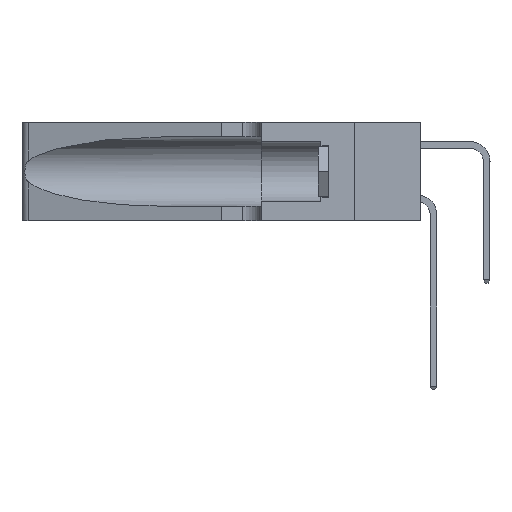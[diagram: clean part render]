
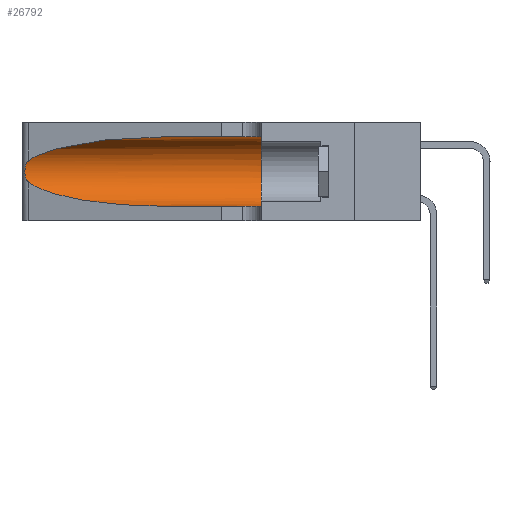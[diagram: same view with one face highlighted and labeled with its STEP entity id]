
A CAD part, left-side view. The second image highlights one B-rep face of the part: STEP entity #26792.
In plain terms, the highlighted cylindrical face has radius 3.308 mm (diameter 6.617 mm), a partial arc.
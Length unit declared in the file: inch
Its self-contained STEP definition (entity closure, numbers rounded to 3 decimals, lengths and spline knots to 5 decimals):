
#36 = EDGE_CURVE ( 'NONE', #20641, #6997, #20732, .T. ) ;
#122 =( BOUNDED_CURVE ( )  B_SPLINE_CURVE ( 3, ( #18034, #7715, #28317, #12953 ),
 .UNSPECIFIED., .F., .F. ) 
 B_SPLINE_CURVE_WITH_KNOTS ( ( 4, 4 ),
 ( 1.5708, 2.84003 ),
 .UNSPECIFIED. ) 
 CURVE ( )  GEOMETRIC_REPRESENTATION_ITEM ( )  RATIONAL_B_SPLINE_CURVE ( ( 1., 0.87, 0.87, 1. ) ) 
 REPRESENTATION_ITEM ( '' )  );
#1109 = EDGE_CURVE ( 'NONE', #9916, #9409, #17977, .T. ) ;
#1591 = EDGE_LOOP ( 'NONE', ( #15493, #31226, #11639, #22113, #8481, #32342 ) ) ;
#1994 = EDGE_CURVE ( 'NONE', #9409, #20641, #33409, .T. ) ;
#2234 = CARTESIAN_POINT ( 'NONE',  ( 0.25789, 1.23486, 0.15765 ) ) ;
#2435 = CARTESIAN_POINT ( 'NONE',  ( 0.1305, 0.35, 0.05475 ) ) ;
#2819 = EDGE_CURVE ( 'NONE', #10085, #6997, #12145, .T. ) ;
#3328 = CARTESIAN_POINT ( 'NONE',  ( 0.25487, 1.22718, 0.14631 ) ) ;
#3401 = CARTESIAN_POINT ( 'NONE',  ( 0.1305, 0.35, 0.31525 ) ) ;
#4725 = CARTESIAN_POINT ( 'NONE',  ( 0.1305, 1.61858, 0.185 ) ) ;
#4908 = CARTESIAN_POINT ( 'NONE',  ( 0.25555, 1.22993, 0.14849 ) ) ;
#4947 = DIRECTION ( 'NONE',  ( 0., -1., 0. ) ) ;
#5436 = CARTESIAN_POINT ( 'NONE',  ( 0.1305, 1.61858, 0.05475 ) ) ;
#6997 = VERTEX_POINT ( 'NONE', #2435 ) ;
#7444 = CARTESIAN_POINT ( 'NONE',  ( 0.25487, 1.22718, 0.22369 ) ) ;
#7674 = EDGE_CURVE ( 'NONE', #18319, #9916, #122, .T. ) ;
#7715 = CARTESIAN_POINT ( 'NONE',  ( 0.18966, 0.96281, 0.31525 ) ) ;
#8481 = ORIENTED_EDGE ( 'NONE', *, *, #2819, .F. ) ;
#9409 = VERTEX_POINT ( 'NONE', #3328 ) ;
#9916 = VERTEX_POINT ( 'NONE', #18435 ) ;
#10061 = CARTESIAN_POINT ( 'NONE',  ( 0.25787, 1.23484, 0.2124 ) ) ;
#10085 = VERTEX_POINT ( 'NONE', #3401 ) ;
#11027 = CARTESIAN_POINT ( 'NONE',  ( 0.1305, 0.72297, 0.05475 ) ) ;
#11028 = CARTESIAN_POINT ( 'NONE',  ( 0.1305, 0.72297, 0.31525 ) ) ;
#11545 = CARTESIAN_POINT ( 'NONE',  ( 0.1305, 0.35, 0.185 ) ) ;
#11639 = ORIENTED_EDGE ( 'NONE', *, *, #1994, .T. ) ;
#12145 = CIRCLE ( 'NONE', #23350, 0.13025 ) ;
#12677 = CARTESIAN_POINT ( 'NONE',  ( 0.26018, 1.23835, 0.19895 ) ) ;
#12953 = CARTESIAN_POINT ( 'NONE',  ( 0.25487, 1.22718, 0.22369 ) ) ;
#13064 = VECTOR ( 'NONE', #20957, 39.37008 ) ;
#13529 = CARTESIAN_POINT ( 'NONE',  ( 0.2373, 1.15595, 0.08982 ) ) ;
#13927 = FACE_OUTER_BOUND ( 'NONE', #1591, .T. ) ;
#14157 = DIRECTION ( 'NONE',  ( 0., 0., 1. ) ) ;
#15298 = CARTESIAN_POINT ( 'NONE',  ( 0.26075, 1.23896, 0.178 ) ) ;
#15493 = ORIENTED_EDGE ( 'NONE', *, *, #7674, .T. ) ;
#17880 = CARTESIAN_POINT ( 'NONE',  ( 0.25856, 1.23593, 0.16098 ) ) ;
#17977 = B_SPLINE_CURVE_WITH_KNOTS ( 'NONE', 3,
 ( #7444, #22931, #25493, #10061, #28051, #12677, #30612, #15298, #33179, #17880, #2234, #20456, #4908, #23040 ),
 .UNSPECIFIED., .F., .F.,
 ( 4, 2, 2, 2, 2, 2, 4 ),
 ( 0., 0.00027, 0.00053, 0.00107, 0.0016, 0.00187, 0.00214 ),
 .UNSPECIFIED. ) ;
#18034 = CARTESIAN_POINT ( 'NONE',  ( 0.1305, 0.72297, 0.31525 ) ) ;
#18319 = VERTEX_POINT ( 'NONE', #11028 ) ;
#18435 = CARTESIAN_POINT ( 'NONE',  ( 0.25487, 1.22718, 0.22369 ) ) ;
#19976 = CYLINDRICAL_SURFACE ( 'NONE', #27251, 0.13025 ) ;
#20155 = DIRECTION ( 'NONE',  ( 0., -1., 0. ) ) ;
#20456 = CARTESIAN_POINT ( 'NONE',  ( 0.25639, 1.23186, 0.15144 ) ) ;
#20641 = VERTEX_POINT ( 'NONE', #25528 ) ;
#20732 = LINE ( 'NONE', #5436, #13064 ) ;
#20957 = DIRECTION ( 'NONE',  ( 0., -1., 0. ) ) ;
#21290 = CARTESIAN_POINT ( 'NONE',  ( 0.25487, 1.22718, 0.14631 ) ) ;
#22113 = ORIENTED_EDGE ( 'NONE', *, *, #36, .T. ) ;
#22931 = CARTESIAN_POINT ( 'NONE',  ( 0.25555, 1.22994, 0.2215 ) ) ;
#22963 = CARTESIAN_POINT ( 'NONE',  ( 0.1305, 1.61858, 0.31525 ) ) ;
#23040 = CARTESIAN_POINT ( 'NONE',  ( 0.25487, 1.22718, 0.14631 ) ) ;
#23350 = AXIS2_PLACEMENT_3D ( 'NONE', #11545, #29506, #14157 ) ;
#25493 = CARTESIAN_POINT ( 'NONE',  ( 0.25639, 1.23184, 0.21858 ) ) ;
#25528 = CARTESIAN_POINT ( 'NONE',  ( 0.1305, 0.72297, 0.05475 ) ) ;
#26428 = CARTESIAN_POINT ( 'NONE',  ( 0.18966, 0.96281, 0.05475 ) ) ;
#26758 = LINE ( 'NONE', #22963, #31931 ) ;
#26792 = ADVANCED_FACE ( 'NONE', ( #13927 ), #19976, .F. ) ;
#26832 = EDGE_CURVE ( 'NONE', #18319, #10085, #26758, .T. ) ;
#27251 = AXIS2_PLACEMENT_3D ( 'NONE', #4725, #20155, #30425 ) ;
#28051 = CARTESIAN_POINT ( 'NONE',  ( 0.25854, 1.2359, 0.20912 ) ) ;
#28317 = CARTESIAN_POINT ( 'NONE',  ( 0.2373, 1.15595, 0.28018 ) ) ;
#29506 = DIRECTION ( 'NONE',  ( 0., 1., 0. ) ) ;
#30425 = DIRECTION ( 'NONE',  ( 0., 0., -1. ) ) ;
#30612 = CARTESIAN_POINT ( 'NONE',  ( 0.26075, 1.23896, 0.19203 ) ) ;
#31226 = ORIENTED_EDGE ( 'NONE', *, *, #1109, .T. ) ;
#31931 = VECTOR ( 'NONE', #4947, 39.37008 ) ;
#32342 = ORIENTED_EDGE ( 'NONE', *, *, #26832, .F. ) ;
#33179 = CARTESIAN_POINT ( 'NONE',  ( 0.26017, 1.23833, 0.17102 ) ) ;
#33409 =( BOUNDED_CURVE ( )  B_SPLINE_CURVE ( 3, ( #21290, #13529, #26428, #11027 ),
 .UNSPECIFIED., .F., .F. ) 
 B_SPLINE_CURVE_WITH_KNOTS ( ( 4, 4 ),
 ( 3.44316, 4.71239 ),
 .UNSPECIFIED. ) 
 CURVE ( )  GEOMETRIC_REPRESENTATION_ITEM ( )  RATIONAL_B_SPLINE_CURVE ( ( 1., 0.87, 0.87, 1. ) ) 
 REPRESENTATION_ITEM ( '' )  );
